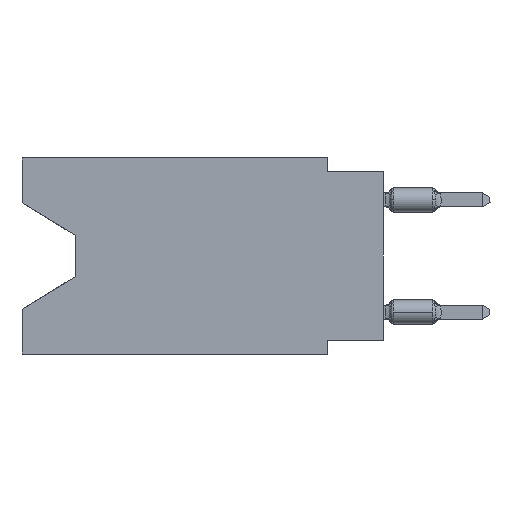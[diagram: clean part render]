
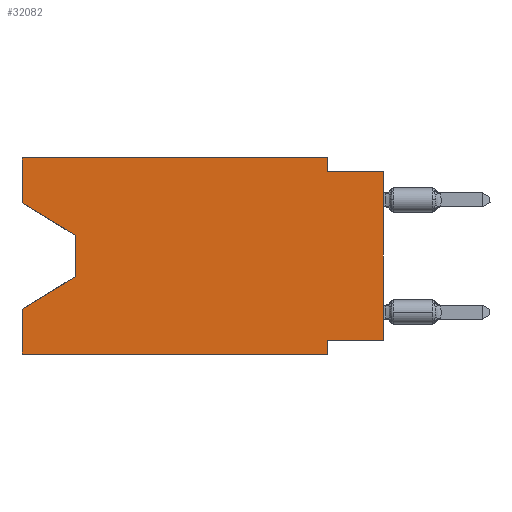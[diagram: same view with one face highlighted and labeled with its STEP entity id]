
A CAD part, left-side view. The second image highlights one B-rep face of the part: STEP entity #32082.
In plain terms, the highlighted planar face has unit normal (-1, 0, 0).
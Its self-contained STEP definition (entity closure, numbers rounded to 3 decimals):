
#163 = LINE ( 'NONE', #24348, #10346 ) ;
#437 = CARTESIAN_POINT ( 'NONE',  ( 0., 13.97, -3.505 ) ) ;
#527 = CARTESIAN_POINT ( 'NONE',  ( 0., 0., 0. ) ) ;
#549 = VERTEX_POINT ( 'NONE', #21637 ) ;
#839 = DIRECTION ( 'NONE',  ( 0., 0., 1. ) ) ;
#1169 = CARTESIAN_POINT ( 'NONE',  ( 0., 16.383, 0. ) ) ;
#1172 = VECTOR ( 'NONE', #21970, 1000. ) ;
#1241 = VERTEX_POINT ( 'NONE', #20986 ) ;
#1474 = EDGE_CURVE ( 'NONE', #19950, #1241, #3856, .T. ) ;
#1565 = LINE ( 'NONE', #33377, #8521 ) ;
#1571 = LINE ( 'NONE', #9853, #1980 ) ;
#1617 = VERTEX_POINT ( 'NONE', #14907 ) ;
#1747 = DIRECTION ( 'NONE',  ( 0., -1., 0. ) ) ;
#1980 = VECTOR ( 'NONE', #1747, 1000. ) ;
#2440 = LINE ( 'NONE', #21628, #9438 ) ;
#2639 = DIRECTION ( 'NONE',  ( 0., 0., 1. ) ) ;
#2996 = LINE ( 'NONE', #18387, #22654 ) ;
#3288 = LINE ( 'NONE', #527, #32975 ) ;
#3815 = EDGE_CURVE ( 'NONE', #32252, #30154, #1565, .T. ) ;
#3840 = CARTESIAN_POINT ( 'NONE',  ( 0., 16.383, 0. ) ) ;
#3856 = LINE ( 'NONE', #29795, #18594 ) ;
#4091 = DIRECTION ( 'NONE',  ( 0., 0., -1. ) ) ;
#4273 = CARTESIAN_POINT ( 'NONE',  ( 0., 16.383, -8.89 ) ) ;
#4319 = ORIENTED_EDGE ( 'NONE', *, *, #6514, .T. ) ;
#4413 = EDGE_LOOP ( 'NONE', ( #4319, #5817, #24709, #24181, #4834, #26580, #31762, #20780, #9106, #6057, #6286, #11724 ) ) ;
#4834 = ORIENTED_EDGE ( 'NONE', *, *, #33742, .T. ) ;
#5607 = EDGE_CURVE ( 'NONE', #17846, #549, #1571, .T. ) ;
#5817 = ORIENTED_EDGE ( 'NONE', *, *, #1474, .T. ) ;
#5961 = CARTESIAN_POINT ( 'NONE',  ( 0., 16.383, -2.038 ) ) ;
#6057 = ORIENTED_EDGE ( 'NONE', *, *, #26182, .F. ) ;
#6141 = CARTESIAN_POINT ( 'NONE',  ( 0., 2.54, -8.255 ) ) ;
#6286 = ORIENTED_EDGE ( 'NONE', *, *, #13918, .F. ) ;
#6514 = EDGE_CURVE ( 'NONE', #28957, #19950, #22646, .T. ) ;
#8298 = CARTESIAN_POINT ( 'NONE',  ( 0., 2.54, -0.635 ) ) ;
#8417 = VERTEX_POINT ( 'NONE', #20692 ) ;
#8521 = VECTOR ( 'NONE', #22650, 1000. ) ;
#8560 = CARTESIAN_POINT ( 'NONE',  ( 0., 0., -8.255 ) ) ;
#8758 = VERTEX_POINT ( 'NONE', #10094 ) ;
#9035 = LINE ( 'NONE', #14565, #20580 ) ;
#9106 = ORIENTED_EDGE ( 'NONE', *, *, #5607, .F. ) ;
#9438 = VECTOR ( 'NONE', #32178, 1000. ) ;
#9853 = CARTESIAN_POINT ( 'NONE',  ( 0., 0., -0.635 ) ) ;
#10094 = CARTESIAN_POINT ( 'NONE',  ( 0., 2.54, 0. ) ) ;
#10249 = CARTESIAN_POINT ( 'NONE',  ( 0., 16.383, 0. ) ) ;
#10346 = VECTOR ( 'NONE', #839, 1000. ) ;
#10574 = FACE_OUTER_BOUND ( 'NONE', #4413, .T. ) ;
#11724 = ORIENTED_EDGE ( 'NONE', *, *, #31355, .F. ) ;
#11796 = DIRECTION ( 'NONE',  ( 0., 0., -1. ) ) ;
#13918 = EDGE_CURVE ( 'NONE', #33177, #8758, #27547, .T. ) ;
#14565 = CARTESIAN_POINT ( 'NONE',  ( 0., 2.54, 0. ) ) ;
#14802 = CARTESIAN_POINT ( 'NONE',  ( 0., 2.54, -8.89 ) ) ;
#14907 = CARTESIAN_POINT ( 'NONE',  ( 0., 2.54, -8.89 ) ) ;
#15951 = VECTOR ( 'NONE', #2639, 1000. ) ;
#17238 = LINE ( 'NONE', #14802, #32644 ) ;
#17846 = VERTEX_POINT ( 'NONE', #8298 ) ;
#18009 = PLANE ( 'NONE',  #32476 ) ;
#18387 = CARTESIAN_POINT ( 'NONE',  ( 0., 16.383, -8.89 ) ) ;
#18594 = VECTOR ( 'NONE', #25139, 1000. ) ;
#19950 = VERTEX_POINT ( 'NONE', #437 ) ;
#20359 = EDGE_CURVE ( 'NONE', #30154, #1617, #17238, .T. ) ;
#20580 = VECTOR ( 'NONE', #11796, 1000. ) ;
#20692 = CARTESIAN_POINT ( 'NONE',  ( 0., 16.383, -6.852 ) ) ;
#20780 = ORIENTED_EDGE ( 'NONE', *, *, #30942, .T. ) ;
#20986 = CARTESIAN_POINT ( 'NONE',  ( 0., 13.97, -5.385 ) ) ;
#21212 = VERTEX_POINT ( 'NONE', #4273 ) ;
#21628 = CARTESIAN_POINT ( 'NONE',  ( 0., 13.97, -5.385 ) ) ;
#21637 = CARTESIAN_POINT ( 'NONE',  ( 0., 0., -0.635 ) ) ;
#21809 = EDGE_CURVE ( 'NONE', #1241, #8417, #2440, .T. ) ;
#21970 = DIRECTION ( 'NONE',  ( 0., -0.855, -0.519 ) ) ;
#22520 = DIRECTION ( 'NONE',  ( 0., -1., 0. ) ) ;
#22646 = LINE ( 'NONE', #25411, #1172 ) ;
#22650 = DIRECTION ( 'NONE',  ( 0., 1., 0. ) ) ;
#22654 = VECTOR ( 'NONE', #31700, 1000. ) ;
#24181 = ORIENTED_EDGE ( 'NONE', *, *, #24822, .F. ) ;
#24348 = CARTESIAN_POINT ( 'NONE',  ( 0., 16.383, 0. ) ) ;
#24385 = DIRECTION ( 'NONE',  ( 0., 0., 1. ) ) ;
#24709 = ORIENTED_EDGE ( 'NONE', *, *, #21809, .T. ) ;
#24822 = EDGE_CURVE ( 'NONE', #21212, #8417, #33940, .T. ) ;
#25139 = DIRECTION ( 'NONE',  ( 0., 0., -1. ) ) ;
#25411 = CARTESIAN_POINT ( 'NONE',  ( 0., 16.383, -2.038 ) ) ;
#25962 = DIRECTION ( 'NONE',  ( 1., 0., 0. ) ) ;
#26182 = EDGE_CURVE ( 'NONE', #8758, #17846, #9035, .T. ) ;
#26580 = ORIENTED_EDGE ( 'NONE', *, *, #20359, .F. ) ;
#27547 = LINE ( 'NONE', #3840, #33856 ) ;
#28556 = CARTESIAN_POINT ( 'NONE',  ( 0., 16.383, 0. ) ) ;
#28957 = VERTEX_POINT ( 'NONE', #5961 ) ;
#29795 = CARTESIAN_POINT ( 'NONE',  ( 0., 13.97, -3.505 ) ) ;
#30154 = VERTEX_POINT ( 'NONE', #6141 ) ;
#30942 = EDGE_CURVE ( 'NONE', #32252, #549, #3288, .T. ) ;
#31355 = EDGE_CURVE ( 'NONE', #28957, #33177, #163, .T. ) ;
#31700 = DIRECTION ( 'NONE',  ( 0., -1., 0. ) ) ;
#31762 = ORIENTED_EDGE ( 'NONE', *, *, #3815, .F. ) ;
#32082 = ADVANCED_FACE ( 'NONE', ( #10574 ), #18009, .F. ) ;
#32178 = DIRECTION ( 'NONE',  ( 0., 0.855, -0.519 ) ) ;
#32252 = VERTEX_POINT ( 'NONE', #8560 ) ;
#32476 = AXIS2_PLACEMENT_3D ( 'NONE', #28556, #25962, #33916 ) ;
#32644 = VECTOR ( 'NONE', #4091, 1000. ) ;
#32975 = VECTOR ( 'NONE', #24385, 1000. ) ;
#33177 = VERTEX_POINT ( 'NONE', #1169 ) ;
#33377 = CARTESIAN_POINT ( 'NONE',  ( 0., 0., -8.255 ) ) ;
#33742 = EDGE_CURVE ( 'NONE', #21212, #1617, #2996, .T. ) ;
#33856 = VECTOR ( 'NONE', #22520, 1000. ) ;
#33916 = DIRECTION ( 'NONE',  ( 0., 0., -1. ) ) ;
#33940 = LINE ( 'NONE', #10249, #15951 ) ;
